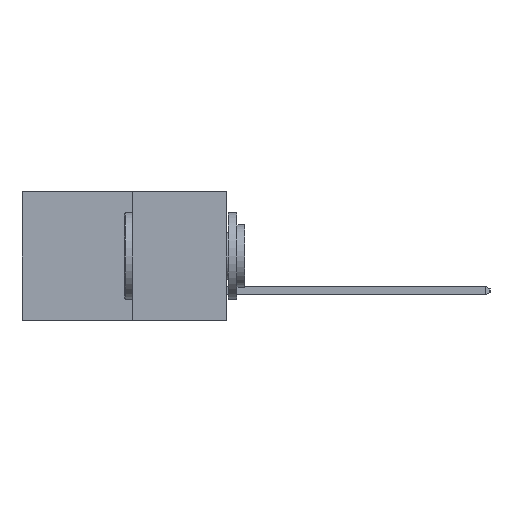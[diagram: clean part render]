
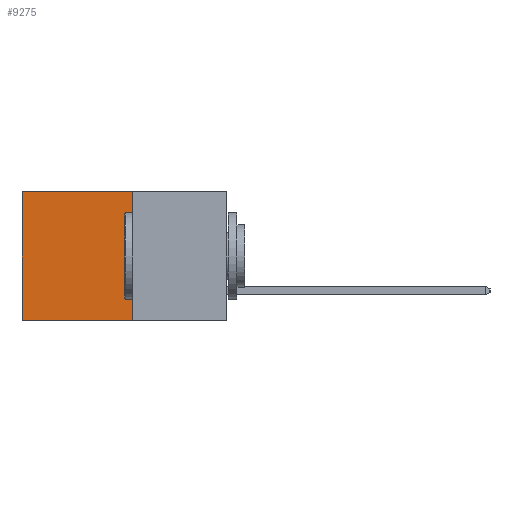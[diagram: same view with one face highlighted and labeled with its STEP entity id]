
A CAD part, left-side view. The second image highlights one B-rep face of the part: STEP entity #9275.
In plain terms, the highlighted planar face has unit normal (-1, 0, 0).
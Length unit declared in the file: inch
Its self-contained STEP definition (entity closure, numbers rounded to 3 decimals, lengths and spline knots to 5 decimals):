
#157 = VERTEX_POINT ( 'NONE', #1386 ) ;
#220 = EDGE_CURVE ( 'NONE', #3077, #2797, #1512, .T. ) ;
#748 = ORIENTED_EDGE ( 'NONE', *, *, #220, .T. ) ;
#1002 = LINE ( 'NONE', #7951, #9857 ) ;
#1057 = ORIENTED_EDGE ( 'NONE', *, *, #10537, .T. ) ;
#1085 = CARTESIAN_POINT ( 'NONE',  ( 0.277, 0.27, -0.37 ) ) ;
#1171 = DIRECTION ( 'NONE',  ( 0., 1., 0. ) ) ;
#1291 = ORIENTED_EDGE ( 'NONE', *, *, #5168, .F. ) ;
#1386 = CARTESIAN_POINT ( 'NONE',  ( 0.277, 0.27, 0. ) ) ;
#1417 = ORIENTED_EDGE ( 'NONE', *, *, #7695, .F. ) ;
#1512 = LINE ( 'NONE', #8860, #3243 ) ;
#2797 = VERTEX_POINT ( 'NONE', #9063 ) ;
#3077 = VERTEX_POINT ( 'NONE', #4474 ) ;
#3243 = VECTOR ( 'NONE', #6448, 39.37008 ) ;
#3765 = CARTESIAN_POINT ( 'NONE',  ( 0.277, 0.27, -0.37 ) ) ;
#3946 = DIRECTION ( 'NONE',  ( 0., 1., 0. ) ) ;
#3994 = CARTESIAN_POINT ( 'NONE',  ( 0.277, 0.27, -0.37 ) ) ;
#4474 = CARTESIAN_POINT ( 'NONE',  ( 0.277, 0.59, 0. ) ) ;
#4654 = DIRECTION ( 'NONE',  ( 0., 0., -1. ) ) ;
#5168 = EDGE_CURVE ( 'NONE', #157, #7375, #1002, .T. ) ;
#5748 = VECTOR ( 'NONE', #1171, 39.37008 ) ;
#6003 = LINE ( 'NONE', #7042, #5748 ) ;
#6411 = VECTOR ( 'NONE', #3946, 39.37008 ) ;
#6448 = DIRECTION ( 'NONE',  ( 0., 0., -1. ) ) ;
#7042 = CARTESIAN_POINT ( 'NONE',  ( 0.277, 0.27, 0. ) ) ;
#7375 = VERTEX_POINT ( 'NONE', #1085 ) ;
#7695 = EDGE_CURVE ( 'NONE', #7375, #2797, #10432, .T. ) ;
#7951 = CARTESIAN_POINT ( 'NONE',  ( 0.277, 0.27, -0.37 ) ) ;
#8628 = EDGE_LOOP ( 'NONE', ( #748, #1417, #1291, #1057 ) ) ;
#8686 = PLANE ( 'NONE',  #9477 ) ;
#8860 = CARTESIAN_POINT ( 'NONE',  ( 0.277, 0.59, -0.37 ) ) ;
#9063 = CARTESIAN_POINT ( 'NONE',  ( 0.277, 0.59, -0.37 ) ) ;
#9275 = ADVANCED_FACE ( 'NONE', ( #9777 ), #8686, .F. ) ;
#9471 = DIRECTION ( 'NONE',  ( 1., 0., 0. ) ) ;
#9477 = AXIS2_PLACEMENT_3D ( 'NONE', #3765, #9471, #4654 ) ;
#9777 = FACE_OUTER_BOUND ( 'NONE', #8628, .T. ) ;
#9857 = VECTOR ( 'NONE', #10657, 39.37008 ) ;
#10432 = LINE ( 'NONE', #3994, #6411 ) ;
#10537 = EDGE_CURVE ( 'NONE', #157, #3077, #6003, .T. ) ;
#10657 = DIRECTION ( 'NONE',  ( 0., 0., -1. ) ) ;
